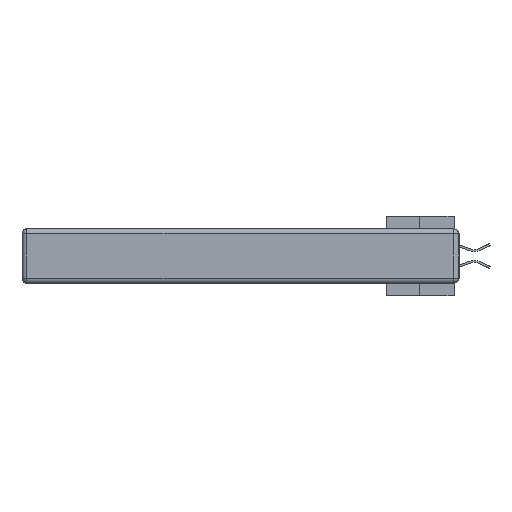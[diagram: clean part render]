
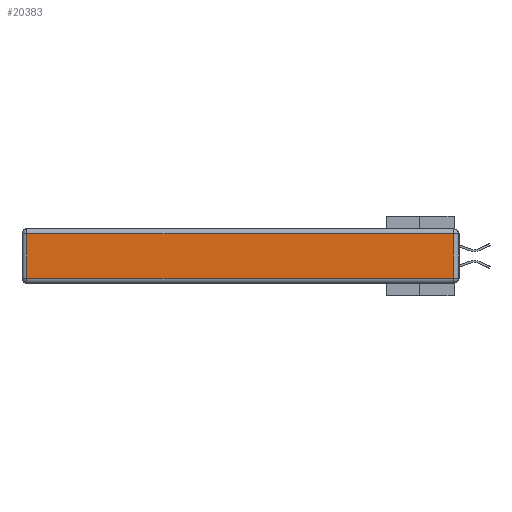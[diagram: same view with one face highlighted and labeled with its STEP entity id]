
A CAD part, left-side view. The second image highlights one B-rep face of the part: STEP entity #20383.
In plain terms, the highlighted planar face has unit normal (-1, 0, 0).
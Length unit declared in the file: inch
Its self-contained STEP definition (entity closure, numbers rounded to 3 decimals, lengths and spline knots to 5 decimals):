
#349 = CARTESIAN_POINT ( 'NONE',  ( 0., 0., -0.313 ) ) ;
#1040 = CARTESIAN_POINT ( 'NONE',  ( 0., 2.72, -0.03 ) ) ;
#1277 = CARTESIAN_POINT ( 'NONE',  ( 0., 0., -0.343 ) ) ;
#4074 = LINE ( 'NONE', #23344, #19793 ) ;
#6110 = FACE_OUTER_BOUND ( 'NONE', #13119, .T. ) ;
#6279 = ORIENTED_EDGE ( 'NONE', *, *, #21927, .T. ) ;
#7717 = PLANE ( 'NONE',  #37087 ) ;
#8220 = VECTOR ( 'NONE', #14634, 39.37008 ) ;
#8972 = CARTESIAN_POINT ( 'NONE',  ( 0., 2.72, -0.313 ) ) ;
#9425 = ORIENTED_EDGE ( 'NONE', *, *, #27503, .T. ) ;
#9709 = VERTEX_POINT ( 'NONE', #8972 ) ;
#11144 = LINE ( 'NONE', #17748, #8220 ) ;
#13119 = EDGE_LOOP ( 'NONE', ( #20621, #9425, #6279, #28454 ) ) ;
#14634 = DIRECTION ( 'NONE',  ( 0., 0., -1. ) ) ;
#17748 = CARTESIAN_POINT ( 'NONE',  ( 0., 2.72, -0.343 ) ) ;
#18871 = LINE ( 'NONE', #349, #25735 ) ;
#19313 = VERTEX_POINT ( 'NONE', #37645 ) ;
#19793 = VECTOR ( 'NONE', #20061, 39.37008 ) ;
#20061 = DIRECTION ( 'NONE',  ( 0., 1., 0. ) ) ;
#20383 = ADVANCED_FACE ( 'NONE', ( #6110 ), #7717, .T. ) ;
#20621 = ORIENTED_EDGE ( 'NONE', *, *, #37883, .T. ) ;
#21927 = EDGE_CURVE ( 'NONE', #19313, #35621, #4074, .T. ) ;
#22143 = CARTESIAN_POINT ( 'NONE',  ( 0., 0.03, -0.343 ) ) ;
#23344 = CARTESIAN_POINT ( 'NONE',  ( 0., 2.75, -0.03 ) ) ;
#25735 = VECTOR ( 'NONE', #31739, 39.37008 ) ;
#26596 = EDGE_CURVE ( 'NONE', #35621, #9709, #11144, .T. ) ;
#27503 = EDGE_CURVE ( 'NONE', #35079, #19313, #39676, .T. ) ;
#28343 = DIRECTION ( 'NONE',  ( 0., 0., 1. ) ) ;
#28454 = ORIENTED_EDGE ( 'NONE', *, *, #26596, .T. ) ;
#31739 = DIRECTION ( 'NONE',  ( 0., -1., 0. ) ) ;
#35079 = VERTEX_POINT ( 'NONE', #36322 ) ;
#35621 = VERTEX_POINT ( 'NONE', #1040 ) ;
#36191 = DIRECTION ( 'NONE',  ( 0., 0., 1. ) ) ;
#36322 = CARTESIAN_POINT ( 'NONE',  ( 0., 0.03, -0.313 ) ) ;
#36713 = VECTOR ( 'NONE', #28343, 39.37008 ) ;
#37087 = AXIS2_PLACEMENT_3D ( 'NONE', #1277, #39345, #36191 ) ;
#37645 = CARTESIAN_POINT ( 'NONE',  ( 0., 0.03, -0.03 ) ) ;
#37883 = EDGE_CURVE ( 'NONE', #9709, #35079, #18871, .T. ) ;
#39345 = DIRECTION ( 'NONE',  ( -1., 0., 0. ) ) ;
#39676 = LINE ( 'NONE', #22143, #36713 ) ;
